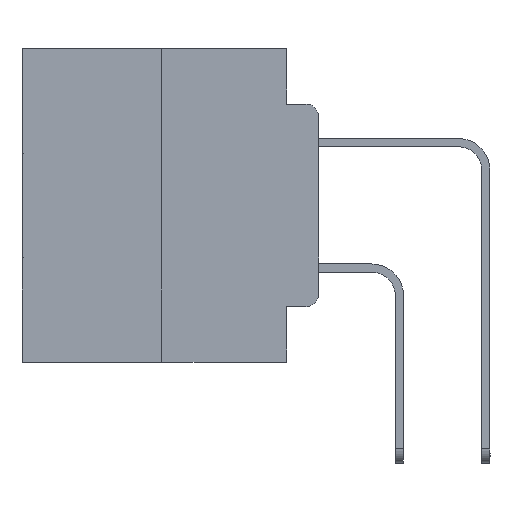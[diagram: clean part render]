
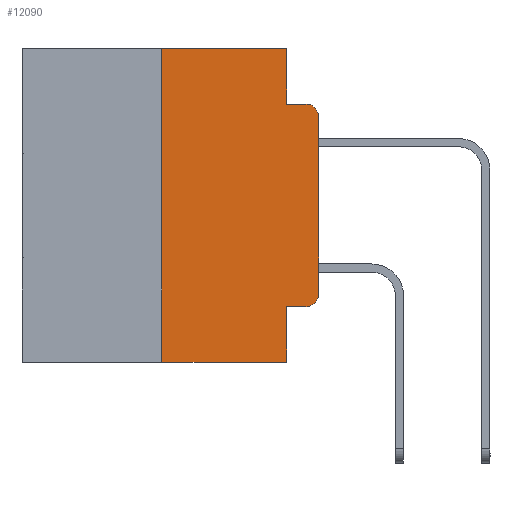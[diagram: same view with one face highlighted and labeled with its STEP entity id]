
A CAD part, left-side view. The second image highlights one B-rep face of the part: STEP entity #12090.
In plain terms, the highlighted planar face has unit normal (-1, 0, 0).
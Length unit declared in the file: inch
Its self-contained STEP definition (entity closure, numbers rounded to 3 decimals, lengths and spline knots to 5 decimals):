
#446 = VECTOR ( 'NONE', #5406, 39.37008 ) ;
#532 = AXIS2_PLACEMENT_3D ( 'NONE', #10198, #15287, #10492 ) ;
#749 = CARTESIAN_POINT ( 'NONE',  ( 0., 0., -0.3915 ) ) ;
#1245 = CARTESIAN_POINT ( 'NONE',  ( 0., 0.473, 0. ) ) ;
#1344 = DIRECTION ( 'NONE',  ( 1., 0., 0. ) ) ;
#1411 = LINE ( 'NONE', #2437, #3229 ) ;
#1863 = LINE ( 'NONE', #13567, #9587 ) ;
#2124 = ORIENTED_EDGE ( 'NONE', *, *, #11311, .F. ) ;
#2437 = CARTESIAN_POINT ( 'NONE',  ( 0., 0.473, 0. ) ) ;
#3180 = DIRECTION ( 'NONE',  ( 0., 0., -1. ) ) ;
#3229 = VECTOR ( 'NONE', #28455, 39.37008 ) ;
#3778 = LINE ( 'NONE', #15585, #7472 ) ;
#4012 = DIRECTION ( 'NONE',  ( 0., 0., 1. ) ) ;
#4167 = VERTEX_POINT ( 'NONE', #27573 ) ;
#4705 = ORIENTED_EDGE ( 'NONE', *, *, #26411, .T. ) ;
#5365 = AXIS2_PLACEMENT_3D ( 'NONE', #28532, #14485, #21166 ) ;
#5406 = DIRECTION ( 'NONE',  ( 0., 0., -1. ) ) ;
#5475 = LINE ( 'NONE', #12412, #16820 ) ;
#5496 = CARTESIAN_POINT ( 'NONE',  ( 0., 0.051, -0.0885 ) ) ;
#6483 = DIRECTION ( 'NONE',  ( 0., 0., 1. ) ) ;
#7472 = VECTOR ( 'NONE', #18343, 39.37008 ) ;
#7520 = EDGE_CURVE ( 'NONE', #20223, #13707, #12655, .T. ) ;
#7865 = CARTESIAN_POINT ( 'NONE',  ( 0., 0.02, -0.4115 ) ) ;
#7941 = CARTESIAN_POINT ( 'NONE',  ( 0., 0.25, 0. ) ) ;
#8966 = DIRECTION ( 'NONE',  ( 0., -1., 0. ) ) ;
#9125 = EDGE_CURVE ( 'NONE', #26256, #20223, #14738, .T. ) ;
#9173 = ORIENTED_EDGE ( 'NONE', *, *, #20472, .T. ) ;
#9223 = VERTEX_POINT ( 'NONE', #7865 ) ;
#9587 = VECTOR ( 'NONE', #8966, 39.37008 ) ;
#9745 = ORIENTED_EDGE ( 'NONE', *, *, #22688, .T. ) ;
#10086 = EDGE_CURVE ( 'NONE', #21798, #17922, #23114, .T. ) ;
#10125 = VECTOR ( 'NONE', #12253, 39.37008 ) ;
#10198 = CARTESIAN_POINT ( 'NONE',  ( 0., 0.02, -0.3915 ) ) ;
#10479 = PLANE ( 'NONE',  #27938 ) ;
#10492 = DIRECTION ( 'NONE',  ( 0., 0., -1. ) ) ;
#10592 = CIRCLE ( 'NONE', #5365, 0.02 ) ;
#10821 = VERTEX_POINT ( 'NONE', #23496 ) ;
#10898 = CARTESIAN_POINT ( 'NONE',  ( 0., 0.25, 0. ) ) ;
#11311 = EDGE_CURVE ( 'NONE', #4167, #10821, #5475, .T. ) ;
#11415 = EDGE_CURVE ( 'NONE', #12939, #13707, #10592, .T. ) ;
#11779 = VECTOR ( 'NONE', #6483, 39.37008 ) ;
#11977 = LINE ( 'NONE', #27284, #24063 ) ;
#12090 = ADVANCED_FACE ( 'NONE', ( #22265 ), #10479, .F. ) ;
#12253 = DIRECTION ( 'NONE',  ( 0., -1., 0. ) ) ;
#12412 = CARTESIAN_POINT ( 'NONE',  ( 0., 0.051, 0. ) ) ;
#12655 = LINE ( 'NONE', #28857, #10125 ) ;
#12939 = VERTEX_POINT ( 'NONE', #19980 ) ;
#13567 = CARTESIAN_POINT ( 'NONE',  ( 0., 0.473, -0.5 ) ) ;
#13707 = VERTEX_POINT ( 'NONE', #24120 ) ;
#13928 = ORIENTED_EDGE ( 'NONE', *, *, #10086, .F. ) ;
#13980 = CARTESIAN_POINT ( 'NONE',  ( 0., 0.051, 0. ) ) ;
#14485 = DIRECTION ( 'NONE',  ( -1., 0., 0. ) ) ;
#14738 = LINE ( 'NONE', #19122, #446 ) ;
#15287 = DIRECTION ( 'NONE',  ( -1., 0., 0. ) ) ;
#15585 = CARTESIAN_POINT ( 'NONE',  ( 0., 0.051, -0.4115 ) ) ;
#16820 = VECTOR ( 'NONE', #3180, 39.37008 ) ;
#17922 = VERTEX_POINT ( 'NONE', #7941 ) ;
#18343 = DIRECTION ( 'NONE',  ( 0., -1., 0. ) ) ;
#19122 = CARTESIAN_POINT ( 'NONE',  ( 0., 0.051, 0. ) ) ;
#19980 = CARTESIAN_POINT ( 'NONE',  ( 0., 0., -0.1085 ) ) ;
#20223 = VERTEX_POINT ( 'NONE', #5496 ) ;
#20472 = EDGE_CURVE ( 'NONE', #21798, #10821, #1863, .T. ) ;
#20486 = ORIENTED_EDGE ( 'NONE', *, *, #27524, .F. ) ;
#21166 = DIRECTION ( 'NONE',  ( 0., 0., -1. ) ) ;
#21403 = ORIENTED_EDGE ( 'NONE', *, *, #24690, .T. ) ;
#21798 = VERTEX_POINT ( 'NONE', #25377 ) ;
#22265 = FACE_OUTER_BOUND ( 'NONE', #26489, .T. ) ;
#22688 = EDGE_CURVE ( 'NONE', #29601, #12939, #11977, .T. ) ;
#23114 = LINE ( 'NONE', #10898, #11779 ) ;
#23496 = CARTESIAN_POINT ( 'NONE',  ( 0., 0.051, -0.5 ) ) ;
#24063 = VECTOR ( 'NONE', #4012, 39.37008 ) ;
#24120 = CARTESIAN_POINT ( 'NONE',  ( 0., 0.02, -0.0885 ) ) ;
#24690 = EDGE_CURVE ( 'NONE', #4167, #9223, #3778, .T. ) ;
#25259 = CIRCLE ( 'NONE', #532, 0.02 ) ;
#25377 = CARTESIAN_POINT ( 'NONE',  ( 0., 0.25, -0.5 ) ) ;
#25736 = ORIENTED_EDGE ( 'NONE', *, *, #9125, .F. ) ;
#26256 = VERTEX_POINT ( 'NONE', #13980 ) ;
#26411 = EDGE_CURVE ( 'NONE', #9223, #29601, #25259, .T. ) ;
#26489 = EDGE_LOOP ( 'NONE', ( #9745, #28764, #29325, #25736, #20486, #13928, #9173, #2124, #21403, #4705 ) ) ;
#26969 = DIRECTION ( 'NONE',  ( 0., 0., -1. ) ) ;
#27284 = CARTESIAN_POINT ( 'NONE',  ( 0., 0., 0. ) ) ;
#27524 = EDGE_CURVE ( 'NONE', #17922, #26256, #1411, .T. ) ;
#27573 = CARTESIAN_POINT ( 'NONE',  ( 0., 0.051, -0.4115 ) ) ;
#27938 = AXIS2_PLACEMENT_3D ( 'NONE', #1245, #1344, #26969 ) ;
#28455 = DIRECTION ( 'NONE',  ( 0., -1., 0. ) ) ;
#28532 = CARTESIAN_POINT ( 'NONE',  ( 0., 0.02, -0.1085 ) ) ;
#28764 = ORIENTED_EDGE ( 'NONE', *, *, #11415, .T. ) ;
#28857 = CARTESIAN_POINT ( 'NONE',  ( 0., 0.051, -0.0885 ) ) ;
#29325 = ORIENTED_EDGE ( 'NONE', *, *, #7520, .F. ) ;
#29601 = VERTEX_POINT ( 'NONE', #749 ) ;
